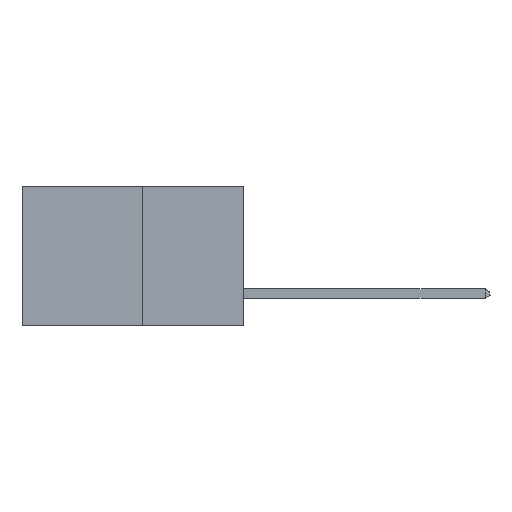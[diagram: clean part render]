
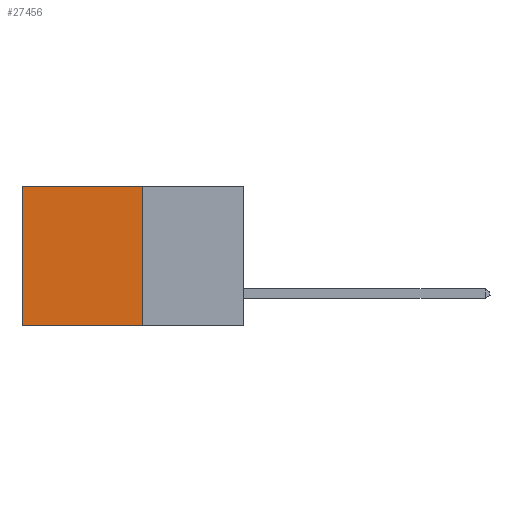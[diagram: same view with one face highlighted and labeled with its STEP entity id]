
A CAD part, left-side view. The second image highlights one B-rep face of the part: STEP entity #27456.
In plain terms, the highlighted planar face has unit normal (-1, 0, 0).
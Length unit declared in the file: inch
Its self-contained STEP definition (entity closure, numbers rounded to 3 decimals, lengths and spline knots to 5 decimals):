
#674 = DIRECTION ( 'NONE',  ( 0., 0., -1. ) ) ;
#892 = VECTOR ( 'NONE', #5646, 39.37008 ) ;
#919 = CARTESIAN_POINT ( 'NONE',  ( 0.277, 0.59, -0.37 ) ) ;
#1295 = CARTESIAN_POINT ( 'NONE',  ( 0.277, 0.27, -0.37 ) ) ;
#1818 = ORIENTED_EDGE ( 'NONE', *, *, #29103, .T. ) ;
#1912 = VERTEX_POINT ( 'NONE', #919 ) ;
#2448 = VECTOR ( 'NONE', #2974, 39.37008 ) ;
#2926 = CARTESIAN_POINT ( 'NONE',  ( 0.277, 0.27, -0.37 ) ) ;
#2974 = DIRECTION ( 'NONE',  ( 0., 1., 0. ) ) ;
#3145 = CARTESIAN_POINT ( 'NONE',  ( 0.277, 0.59, 0. ) ) ;
#3799 = DIRECTION ( 'NONE',  ( 1., 0., 0. ) ) ;
#3873 = EDGE_CURVE ( 'NONE', #9021, #1912, #19722, .T. ) ;
#5646 = DIRECTION ( 'NONE',  ( 0., 1., 0. ) ) ;
#6042 = LINE ( 'NONE', #12949, #13322 ) ;
#7126 = FACE_OUTER_BOUND ( 'NONE', #17238, .T. ) ;
#7416 = ORIENTED_EDGE ( 'NONE', *, *, #27659, .T. ) ;
#8232 = ORIENTED_EDGE ( 'NONE', *, *, #3873, .F. ) ;
#9021 = VERTEX_POINT ( 'NONE', #2926 ) ;
#9752 = LINE ( 'NONE', #17801, #2448 ) ;
#12949 = CARTESIAN_POINT ( 'NONE',  ( 0.277, 0.27, -0.37 ) ) ;
#13322 = VECTOR ( 'NONE', #674, 39.37008 ) ;
#13613 = CARTESIAN_POINT ( 'NONE',  ( 0.277, 0.27, 0. ) ) ;
#14016 = LINE ( 'NONE', #17659, #25410 ) ;
#14933 = VERTEX_POINT ( 'NONE', #13613 ) ;
#16054 = PLANE ( 'NONE',  #27736 ) ;
#17238 = EDGE_LOOP ( 'NONE', ( #7416, #8232, #18642, #1818 ) ) ;
#17659 = CARTESIAN_POINT ( 'NONE',  ( 0.277, 0.59, -0.37 ) ) ;
#17801 = CARTESIAN_POINT ( 'NONE',  ( 0.277, 0.27, 0. ) ) ;
#18642 = ORIENTED_EDGE ( 'NONE', *, *, #22480, .F. ) ;
#19722 = LINE ( 'NONE', #20322, #892 ) ;
#20078 = DIRECTION ( 'NONE',  ( 0., 0., -1. ) ) ;
#20322 = CARTESIAN_POINT ( 'NONE',  ( 0.277, 0.27, -0.37 ) ) ;
#20938 = DIRECTION ( 'NONE',  ( 0., 0., -1. ) ) ;
#22480 = EDGE_CURVE ( 'NONE', #14933, #9021, #6042, .T. ) ;
#25410 = VECTOR ( 'NONE', #20078, 39.37008 ) ;
#27456 = ADVANCED_FACE ( 'NONE', ( #7126 ), #16054, .F. ) ;
#27659 = EDGE_CURVE ( 'NONE', #31205, #1912, #14016, .T. ) ;
#27736 = AXIS2_PLACEMENT_3D ( 'NONE', #1295, #3799, #20938 ) ;
#29103 = EDGE_CURVE ( 'NONE', #14933, #31205, #9752, .T. ) ;
#31205 = VERTEX_POINT ( 'NONE', #3145 ) ;
